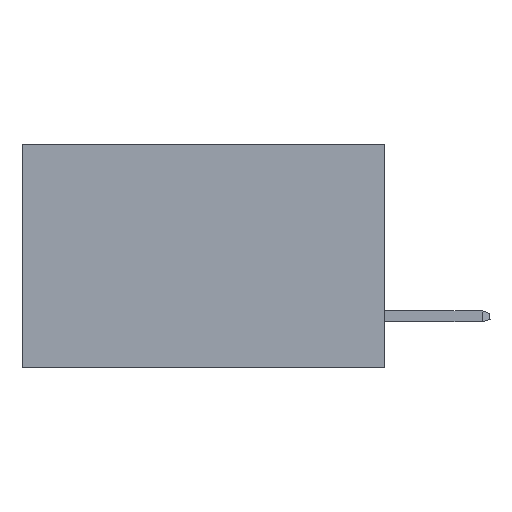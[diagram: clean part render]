
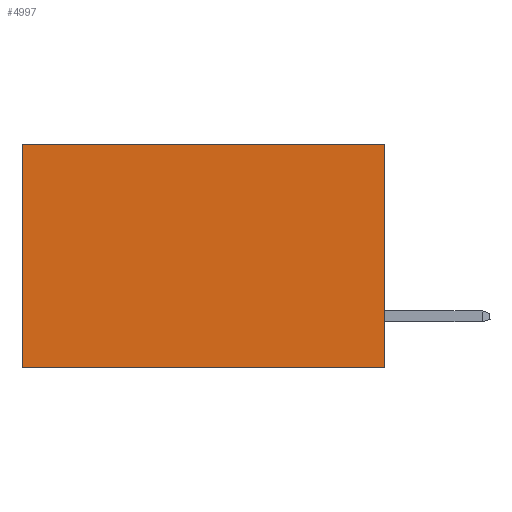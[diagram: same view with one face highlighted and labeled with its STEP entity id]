
A CAD part, left-side view. The second image highlights one B-rep face of the part: STEP entity #4997.
In plain terms, the highlighted planar face has unit normal (-1, 0, 0).
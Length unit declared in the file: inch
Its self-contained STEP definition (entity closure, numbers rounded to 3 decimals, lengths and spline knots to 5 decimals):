
#1250 = VECTOR ( 'NONE', #13562, 39.37008 ) ;
#1768 = VERTEX_POINT ( 'NONE', #5552 ) ;
#2114 = LINE ( 'NONE', #10345, #6284 ) ;
#3895 = EDGE_CURVE ( 'NONE', #10999, #8822, #7751, .T. ) ;
#4997 = ADVANCED_FACE ( 'NONE', ( #29453 ), #25668, .F. ) ;
#5083 = CARTESIAN_POINT ( 'NONE',  ( 0.298, 0., 0. ) ) ;
#5425 = EDGE_LOOP ( 'NONE', ( #23661, #15683, #13141, #31102 ) ) ;
#5552 = CARTESIAN_POINT ( 'NONE',  ( 0.298, 0., -0.37 ) ) ;
#5672 = EDGE_CURVE ( 'NONE', #21098, #10999, #23833, .T. ) ;
#6284 = VECTOR ( 'NONE', #14997, 39.37008 ) ;
#7188 = LINE ( 'NONE', #27803, #28594 ) ;
#7751 = LINE ( 'NONE', #18844, #1250 ) ;
#8822 = VERTEX_POINT ( 'NONE', #16638 ) ;
#10345 = CARTESIAN_POINT ( 'NONE',  ( 0.298, 0., -0.37 ) ) ;
#10918 = DIRECTION ( 'NONE',  ( 0., 0., -1. ) ) ;
#10999 = VERTEX_POINT ( 'NONE', #21618 ) ;
#13141 = ORIENTED_EDGE ( 'NONE', *, *, #21186, .F. ) ;
#13562 = DIRECTION ( 'NONE',  ( 0., 0., -1. ) ) ;
#14089 = DIRECTION ( 'NONE',  ( 0., 0., -1. ) ) ;
#14770 = DIRECTION ( 'NONE',  ( 0., 1., 0. ) ) ;
#14997 = DIRECTION ( 'NONE',  ( 0., 1., 0. ) ) ;
#15683 = ORIENTED_EDGE ( 'NONE', *, *, #23880, .F. ) ;
#16638 = CARTESIAN_POINT ( 'NONE',  ( 0.298, 0.6, -0.37 ) ) ;
#18844 = CARTESIAN_POINT ( 'NONE',  ( 0.298, 0.6, 0. ) ) ;
#21098 = VERTEX_POINT ( 'NONE', #5083 ) ;
#21186 = EDGE_CURVE ( 'NONE', #21098, #1768, #7188, .T. ) ;
#21618 = CARTESIAN_POINT ( 'NONE',  ( 0.298, 0.6, 0. ) ) ;
#23625 = CARTESIAN_POINT ( 'NONE',  ( 0.298, 0., 0. ) ) ;
#23661 = ORIENTED_EDGE ( 'NONE', *, *, #3895, .T. ) ;
#23833 = LINE ( 'NONE', #26803, #28334 ) ;
#23880 = EDGE_CURVE ( 'NONE', #1768, #8822, #2114, .T. ) ;
#25668 = PLANE ( 'NONE',  #30606 ) ;
#26803 = CARTESIAN_POINT ( 'NONE',  ( 0.298, 0., 0. ) ) ;
#27803 = CARTESIAN_POINT ( 'NONE',  ( 0.298, 0., 0. ) ) ;
#28334 = VECTOR ( 'NONE', #14770, 39.37008 ) ;
#28547 = DIRECTION ( 'NONE',  ( 1., 0., 0. ) ) ;
#28594 = VECTOR ( 'NONE', #10918, 39.37008 ) ;
#29453 = FACE_OUTER_BOUND ( 'NONE', #5425, .T. ) ;
#30606 = AXIS2_PLACEMENT_3D ( 'NONE', #23625, #28547, #14089 ) ;
#31102 = ORIENTED_EDGE ( 'NONE', *, *, #5672, .T. ) ;
